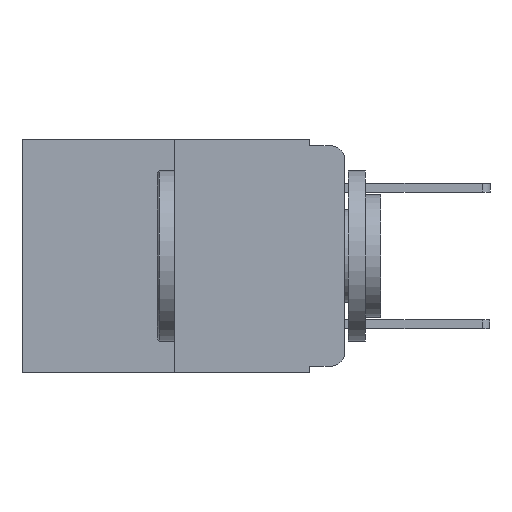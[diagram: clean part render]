
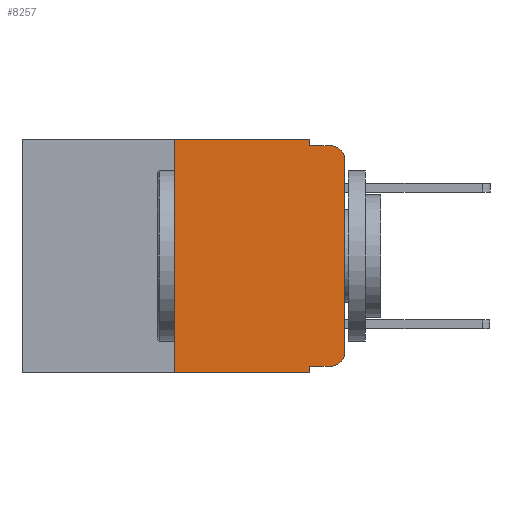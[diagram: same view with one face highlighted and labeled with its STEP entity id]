
A CAD part, left-side view. The second image highlights one B-rep face of the part: STEP entity #8257.
In plain terms, the highlighted planar face has unit normal (-1, 0, 0).
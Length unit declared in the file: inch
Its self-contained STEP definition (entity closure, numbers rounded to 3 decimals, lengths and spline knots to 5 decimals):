
#233 = CIRCLE ( 'NONE', #19883, 0.02 ) ;
#515 = CARTESIAN_POINT ( 'NONE',  ( 0., 0., -0.03 ) ) ;
#662 = VECTOR ( 'NONE', #15030, 39.37008 ) ;
#1153 = DIRECTION ( 'NONE',  ( -1., 0., 0. ) ) ;
#1292 = VERTEX_POINT ( 'NONE', #20183 ) ;
#1546 = CARTESIAN_POINT ( 'NONE',  ( 0., 0.051, 0. ) ) ;
#1780 = FACE_OUTER_BOUND ( 'NONE', #24453, .T. ) ;
#2255 = CARTESIAN_POINT ( 'NONE',  ( 0., 0.25, 0. ) ) ;
#2343 = DIRECTION ( 'NONE',  ( 0., 0., 1. ) ) ;
#2563 = VECTOR ( 'NONE', #20500, 39.37008 ) ;
#2747 = CARTESIAN_POINT ( 'NONE',  ( 0., 0.02, -0.313 ) ) ;
#3049 = VERTEX_POINT ( 'NONE', #9744 ) ;
#3312 = VERTEX_POINT ( 'NONE', #12130 ) ;
#3313 = VERTEX_POINT ( 'NONE', #24420 ) ;
#3338 = EDGE_CURVE ( 'NONE', #6330, #22803, #17300, .T. ) ;
#3354 = CARTESIAN_POINT ( 'NONE',  ( 0., 0.051, -0.01 ) ) ;
#3702 = LINE ( 'NONE', #17319, #18255 ) ;
#4674 = AXIS2_PLACEMENT_3D ( 'NONE', #2747, #16080, #4706 ) ;
#4706 = DIRECTION ( 'NONE',  ( 0., 0., -1. ) ) ;
#5107 = EDGE_CURVE ( 'NONE', #22803, #18619, #14499, .T. ) ;
#5541 = CARTESIAN_POINT ( 'NONE',  ( 0., 0., 0. ) ) ;
#5977 = ORIENTED_EDGE ( 'NONE', *, *, #20624, .T. ) ;
#6189 = DIRECTION ( 'NONE',  ( 0., 0., -1. ) ) ;
#6330 = VERTEX_POINT ( 'NONE', #1546 ) ;
#6510 = LINE ( 'NONE', #5541, #662 ) ;
#7180 = ORIENTED_EDGE ( 'NONE', *, *, #13081, .T. ) ;
#7331 = CARTESIAN_POINT ( 'NONE',  ( 0., 0.473, 0. ) ) ;
#8257 = ADVANCED_FACE ( 'NONE', ( #1780 ), #15643, .F. ) ;
#8517 = CIRCLE ( 'NONE', #4674, 0.02 ) ;
#8786 = DIRECTION ( 'NONE',  ( 0., -1., 0. ) ) ;
#8858 = VECTOR ( 'NONE', #14843, 39.37008 ) ;
#9726 = AXIS2_PLACEMENT_3D ( 'NONE', #11839, #17512, #6189 ) ;
#9744 = CARTESIAN_POINT ( 'NONE',  ( 0., 0.051, -0.343 ) ) ;
#9802 = CARTESIAN_POINT ( 'NONE',  ( 0., 0.051, 0. ) ) ;
#10579 = VECTOR ( 'NONE', #8786, 39.37008 ) ;
#10615 = EDGE_CURVE ( 'NONE', #12881, #6330, #22080, .T. ) ;
#10692 = EDGE_CURVE ( 'NONE', #3313, #21331, #6510, .T. ) ;
#11764 = CARTESIAN_POINT ( 'NONE',  ( 0., 0.051, 0. ) ) ;
#11812 = LINE ( 'NONE', #2255, #15066 ) ;
#11839 = CARTESIAN_POINT ( 'NONE',  ( 0., 0.473, 0. ) ) ;
#12130 = CARTESIAN_POINT ( 'NONE',  ( 0., 0.02, -0.333 ) ) ;
#12519 = CARTESIAN_POINT ( 'NONE',  ( 0., 0.473, -0.343 ) ) ;
#12683 = CARTESIAN_POINT ( 'NONE',  ( 0., 0.02, -0.03 ) ) ;
#12881 = VERTEX_POINT ( 'NONE', #22277 ) ;
#12920 = LINE ( 'NONE', #11764, #22840 ) ;
#13081 = EDGE_CURVE ( 'NONE', #1292, #3312, #3702, .T. ) ;
#13282 = CARTESIAN_POINT ( 'NONE',  ( 0., 0.25, -0.343 ) ) ;
#14122 = ORIENTED_EDGE ( 'NONE', *, *, #21055, .F. ) ;
#14499 = LINE ( 'NONE', #3354, #8858 ) ;
#14593 = DIRECTION ( 'NONE',  ( 0., 0., -1. ) ) ;
#14843 = DIRECTION ( 'NONE',  ( 0., -1., 0. ) ) ;
#15030 = DIRECTION ( 'NONE',  ( 0., 0., 1. ) ) ;
#15066 = VECTOR ( 'NONE', #2343, 39.37008 ) ;
#15643 = PLANE ( 'NONE',  #9726 ) ;
#15860 = VERTEX_POINT ( 'NONE', #13282 ) ;
#15877 = ORIENTED_EDGE ( 'NONE', *, *, #20726, .T. ) ;
#16080 = DIRECTION ( 'NONE',  ( -1., 0., 0. ) ) ;
#16119 = ORIENTED_EDGE ( 'NONE', *, *, #19851, .F. ) ;
#16192 = ORIENTED_EDGE ( 'NONE', *, *, #10615, .F. ) ;
#16205 = LINE ( 'NONE', #12519, #10579 ) ;
#16244 = DIRECTION ( 'NONE',  ( 0., 0., -1. ) ) ;
#16445 = ORIENTED_EDGE ( 'NONE', *, *, #3338, .F. ) ;
#17300 = LINE ( 'NONE', #9802, #22235 ) ;
#17319 = CARTESIAN_POINT ( 'NONE',  ( 0., 0.051, -0.333 ) ) ;
#17512 = DIRECTION ( 'NONE',  ( 1., 0., 0. ) ) ;
#18255 = VECTOR ( 'NONE', #22679, 39.37008 ) ;
#18497 = ORIENTED_EDGE ( 'NONE', *, *, #5107, .F. ) ;
#18619 = VERTEX_POINT ( 'NONE', #19182 ) ;
#18726 = ORIENTED_EDGE ( 'NONE', *, *, #20755, .T. ) ;
#19182 = CARTESIAN_POINT ( 'NONE',  ( 0., 0.02, -0.01 ) ) ;
#19761 = ORIENTED_EDGE ( 'NONE', *, *, #10692, .T. ) ;
#19851 = EDGE_CURVE ( 'NONE', #15860, #12881, #11812, .T. ) ;
#19883 = AXIS2_PLACEMENT_3D ( 'NONE', #12683, #1153, #14593 ) ;
#20183 = CARTESIAN_POINT ( 'NONE',  ( 0., 0.051, -0.333 ) ) ;
#20500 = DIRECTION ( 'NONE',  ( 0., -1., 0. ) ) ;
#20624 = EDGE_CURVE ( 'NONE', #3312, #3313, #8517, .T. ) ;
#20726 = EDGE_CURVE ( 'NONE', #15860, #3049, #16205, .T. ) ;
#20755 = EDGE_CURVE ( 'NONE', #21331, #18619, #233, .T. ) ;
#21055 = EDGE_CURVE ( 'NONE', #1292, #3049, #12920, .T. ) ;
#21331 = VERTEX_POINT ( 'NONE', #515 ) ;
#22080 = LINE ( 'NONE', #7331, #2563 ) ;
#22235 = VECTOR ( 'NONE', #16244, 39.37008 ) ;
#22277 = CARTESIAN_POINT ( 'NONE',  ( 0., 0.25, 0. ) ) ;
#22679 = DIRECTION ( 'NONE',  ( 0., -1., 0. ) ) ;
#22803 = VERTEX_POINT ( 'NONE', #24160 ) ;
#22840 = VECTOR ( 'NONE', #22938, 39.37008 ) ;
#22938 = DIRECTION ( 'NONE',  ( 0., 0., -1. ) ) ;
#24160 = CARTESIAN_POINT ( 'NONE',  ( 0., 0.051, -0.01 ) ) ;
#24420 = CARTESIAN_POINT ( 'NONE',  ( 0., 0., -0.313 ) ) ;
#24453 = EDGE_LOOP ( 'NONE', ( #19761, #18726, #18497, #16445, #16192, #16119, #15877, #14122, #7180, #5977 ) ) ;
